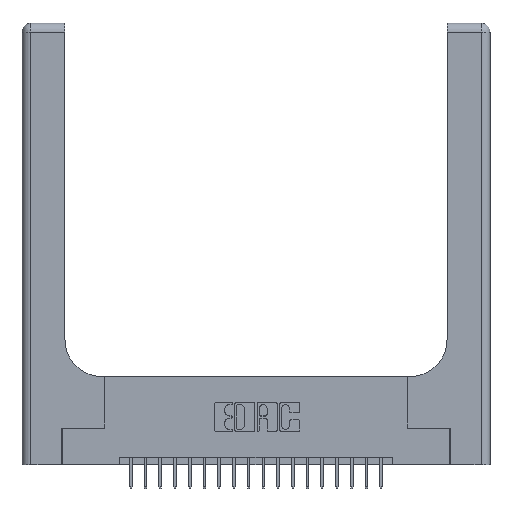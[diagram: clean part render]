
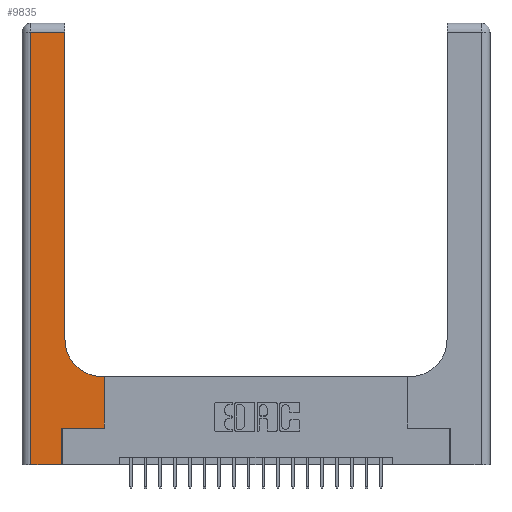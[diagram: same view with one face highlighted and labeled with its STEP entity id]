
A CAD part, top view. The second image highlights one B-rep face of the part: STEP entity #9835.
In plain terms, the highlighted planar face has unit normal (0, 0, 1).
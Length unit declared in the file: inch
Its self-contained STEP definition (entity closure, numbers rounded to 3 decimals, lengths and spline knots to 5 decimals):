
#364 = CARTESIAN_POINT ( 'NONE',  ( 0.5585, 0.25, 0.37 ) ) ;
#836 = VECTOR ( 'NONE', #5833, 39.37008 ) ;
#915 = EDGE_CURVE ( 'NONE', #20956, #6782, #6176, .T. ) ;
#1226 = AXIS2_PLACEMENT_3D ( 'NONE', #18210, #2417, #9261 ) ;
#1649 = ORIENTED_EDGE ( 'NONE', *, *, #11550, .T. ) ;
#1720 = EDGE_CURVE ( 'NONE', #18494, #2396, #20425, .T. ) ;
#1738 = VECTOR ( 'NONE', #14002, 39.37008 ) ;
#2030 = LINE ( 'NONE', #17034, #6158 ) ;
#2396 = VERTEX_POINT ( 'NONE', #13441 ) ;
#2417 = DIRECTION ( 'NONE',  ( 0., 0., -1. ) ) ;
#2759 = CARTESIAN_POINT ( 'NONE',  ( 0.269, 0., 0.37 ) ) ;
#3298 = CIRCLE ( 'NONE', #15200, 0.25 ) ;
#4452 = VECTOR ( 'NONE', #11610, 39.37008 ) ;
#4602 = DIRECTION ( 'NONE',  ( 0., -1., 0. ) ) ;
#4731 = CARTESIAN_POINT ( 'NONE',  ( 0.269, 0.25, 0.37 ) ) ;
#5372 = DIRECTION ( 'NONE',  ( 0., 1., 0. ) ) ;
#5433 = EDGE_CURVE ( 'NONE', #22096, #5551, #9410, .T. ) ;
#5551 = VERTEX_POINT ( 'NONE', #7782 ) ;
#5637 = DIRECTION ( 'NONE',  ( 1., 0., 0. ) ) ;
#5797 = LINE ( 'NONE', #12575, #836 ) ;
#5833 = DIRECTION ( 'NONE',  ( -1., 0., 0. ) ) ;
#5985 = ORIENTED_EDGE ( 'NONE', *, *, #5433, .T. ) ;
#6158 = VECTOR ( 'NONE', #6692, 39.37008 ) ;
#6176 = LINE ( 'NONE', #14384, #12217 ) ;
#6405 = EDGE_CURVE ( 'NONE', #6782, #18494, #5797, .T. ) ;
#6674 = LINE ( 'NONE', #10626, #1738 ) ;
#6692 = DIRECTION ( 'NONE',  ( -1., 0., 0. ) ) ;
#6782 = VERTEX_POINT ( 'NONE', #12481 ) ;
#7105 = VECTOR ( 'NONE', #5637, 39.37008 ) ;
#7200 = VECTOR ( 'NONE', #5372, 39.37008 ) ;
#7649 = PLANE ( 'NONE',  #1226 ) ;
#7782 = CARTESIAN_POINT ( 'NONE',  ( 0.5585, 0.6, 0.37 ) ) ;
#7994 = EDGE_CURVE ( 'NONE', #10890, #22096, #12041, .T. ) ;
#8297 = LINE ( 'NONE', #2759, #4452 ) ;
#8630 = CARTESIAN_POINT ( 'NONE',  ( 0.269, 0., 0.37 ) ) ;
#9261 = DIRECTION ( 'NONE',  ( -1., 0., 0. ) ) ;
#9410 = LINE ( 'NONE', #16100, #7200 ) ;
#9835 = ADVANCED_FACE ( 'NONE', ( #17423 ), #7649, .F. ) ;
#10320 = DIRECTION ( 'NONE',  ( 0., 0., -1. ) ) ;
#10626 = CARTESIAN_POINT ( 'NONE',  ( 0., 0., 0.37 ) ) ;
#10890 = VERTEX_POINT ( 'NONE', #4731 ) ;
#11242 = CARTESIAN_POINT ( 'NONE',  ( 0.5415, 0.6, 0.37 ) ) ;
#11550 = EDGE_CURVE ( 'NONE', #11786, #20956, #3298, .T. ) ;
#11610 = DIRECTION ( 'NONE',  ( 0., 1., 0. ) ) ;
#11666 = ORIENTED_EDGE ( 'NONE', *, *, #7994, .T. ) ;
#11728 = CARTESIAN_POINT ( 'NONE',  ( 0.2915, 0.85, 0.37 ) ) ;
#11786 = VERTEX_POINT ( 'NONE', #11242 ) ;
#11946 = CARTESIAN_POINT ( 'NONE',  ( 0.5415, 0.85, 0.37 ) ) ;
#11964 = VECTOR ( 'NONE', #4602, 39.37008 ) ;
#12041 = LINE ( 'NONE', #15716, #7105 ) ;
#12217 = VECTOR ( 'NONE', #19811, 39.37008 ) ;
#12305 = EDGE_LOOP ( 'NONE', ( #21903, #21512, #13361, #12565, #14180, #11666, #5985, #15678, #1649 ) ) ;
#12481 = CARTESIAN_POINT ( 'NONE',  ( 0.2915, 2.94, 0.37 ) ) ;
#12565 = ORIENTED_EDGE ( 'NONE', *, *, #21267, .T. ) ;
#12575 = CARTESIAN_POINT ( 'NONE',  ( 0., 2.94, 0.37 ) ) ;
#13361 = ORIENTED_EDGE ( 'NONE', *, *, #1720, .T. ) ;
#13441 = CARTESIAN_POINT ( 'NONE',  ( 0.06, 0., 0.37 ) ) ;
#14002 = DIRECTION ( 'NONE',  ( 1., 0., 0. ) ) ;
#14180 = ORIENTED_EDGE ( 'NONE', *, *, #21725, .T. ) ;
#14384 = CARTESIAN_POINT ( 'NONE',  ( 0.2915, 3., 0.37 ) ) ;
#15200 = AXIS2_PLACEMENT_3D ( 'NONE', #11946, #10320, #17137 ) ;
#15678 = ORIENTED_EDGE ( 'NONE', *, *, #16291, .T. ) ;
#15716 = CARTESIAN_POINT ( 'NONE',  ( 0.269, 0.25, 0.37 ) ) ;
#16100 = CARTESIAN_POINT ( 'NONE',  ( 0.5585, 0.25, 0.37 ) ) ;
#16291 = EDGE_CURVE ( 'NONE', #5551, #11786, #2030, .T. ) ;
#17034 = CARTESIAN_POINT ( 'NONE',  ( 0.2915, 0.6, 0.37 ) ) ;
#17137 = DIRECTION ( 'NONE',  ( 1., 0., 0. ) ) ;
#17423 = FACE_OUTER_BOUND ( 'NONE', #12305, .T. ) ;
#18210 = CARTESIAN_POINT ( 'NONE',  ( 0., 3., 0.37 ) ) ;
#18394 = CARTESIAN_POINT ( 'NONE',  ( 0.06, 3., 0.37 ) ) ;
#18494 = VERTEX_POINT ( 'NONE', #19931 ) ;
#19811 = DIRECTION ( 'NONE',  ( 0., 1., 0. ) ) ;
#19931 = CARTESIAN_POINT ( 'NONE',  ( 0.06, 2.94, 0.37 ) ) ;
#20425 = LINE ( 'NONE', #18394, #11964 ) ;
#20956 = VERTEX_POINT ( 'NONE', #11728 ) ;
#21101 = VERTEX_POINT ( 'NONE', #8630 ) ;
#21267 = EDGE_CURVE ( 'NONE', #2396, #21101, #6674, .T. ) ;
#21512 = ORIENTED_EDGE ( 'NONE', *, *, #6405, .T. ) ;
#21725 = EDGE_CURVE ( 'NONE', #21101, #10890, #8297, .T. ) ;
#21903 = ORIENTED_EDGE ( 'NONE', *, *, #915, .T. ) ;
#22096 = VERTEX_POINT ( 'NONE', #364 ) ;
